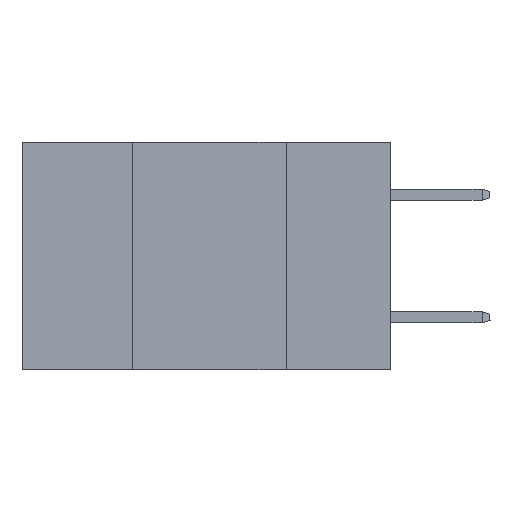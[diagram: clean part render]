
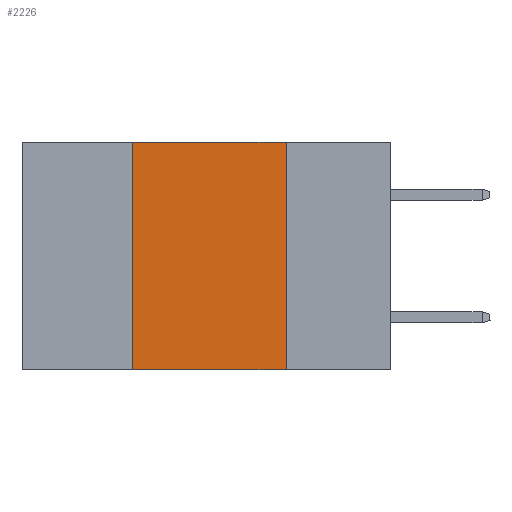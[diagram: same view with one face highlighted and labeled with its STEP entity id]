
A CAD part, left-side view. The second image highlights one B-rep face of the part: STEP entity #2226.
In plain terms, the highlighted planar face has unit normal (-1, 0, 0).
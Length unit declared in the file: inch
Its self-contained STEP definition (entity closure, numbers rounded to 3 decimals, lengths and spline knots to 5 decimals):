
#25 = DIRECTION ( 'NONE',  ( 0., 0., -1. ) ) ;
#101 = VERTEX_POINT ( 'NONE', #484 ) ;
#113 = VERTEX_POINT ( 'NONE', #12711 ) ;
#406 = EDGE_CURVE ( 'NONE', #113, #9413, #10536, .T. ) ;
#484 = CARTESIAN_POINT ( 'NONE',  ( 0., 0.42, -0.37 ) ) ;
#490 = DIRECTION ( 'NONE',  ( 0., 0., 1. ) ) ;
#513 = CARTESIAN_POINT ( 'NONE',  ( 0., 0.42, 0. ) ) ;
#1226 = VECTOR ( 'NONE', #4649, 39.37008 ) ;
#1314 = VECTOR ( 'NONE', #18355, 39.37008 ) ;
#2226 = ADVANCED_FACE ( 'NONE', ( #9738 ), #15655, .F. ) ;
#2980 = EDGE_CURVE ( 'NONE', #7673, #113, #4818, .T. ) ;
#3678 = CARTESIAN_POINT ( 'NONE',  ( 0., 0.6, -0.37 ) ) ;
#4121 = CARTESIAN_POINT ( 'NONE',  ( 0., 0.17, 0. ) ) ;
#4517 = CARTESIAN_POINT ( 'NONE',  ( 0., 0.17, -0.37 ) ) ;
#4649 = DIRECTION ( 'NONE',  ( 0., -1., 0. ) ) ;
#4818 = LINE ( 'NONE', #10713, #1226 ) ;
#5288 = EDGE_LOOP ( 'NONE', ( #19977, #6167, #11014, #10120 ) ) ;
#5918 = VECTOR ( 'NONE', #16476, 39.37008 ) ;
#6167 = ORIENTED_EDGE ( 'NONE', *, *, #2980, .F. ) ;
#7673 = VERTEX_POINT ( 'NONE', #513 ) ;
#7856 = DIRECTION ( 'NONE',  ( 1., 0., 0. ) ) ;
#7920 = CARTESIAN_POINT ( 'NONE',  ( 0., 0.6, 0. ) ) ;
#9349 = AXIS2_PLACEMENT_3D ( 'NONE', #7920, #7856, #25 ) ;
#9413 = VERTEX_POINT ( 'NONE', #4517 ) ;
#9419 = EDGE_CURVE ( 'NONE', #101, #7673, #17375, .T. ) ;
#9507 = CARTESIAN_POINT ( 'NONE',  ( 0., 0.42, 0. ) ) ;
#9738 = FACE_OUTER_BOUND ( 'NONE', #5288, .T. ) ;
#10120 = ORIENTED_EDGE ( 'NONE', *, *, #15979, .T. ) ;
#10536 = LINE ( 'NONE', #4121, #5918 ) ;
#10713 = CARTESIAN_POINT ( 'NONE',  ( 0., 0.6, 0. ) ) ;
#11014 = ORIENTED_EDGE ( 'NONE', *, *, #9419, .F. ) ;
#12219 = VECTOR ( 'NONE', #490, 39.37008 ) ;
#12711 = CARTESIAN_POINT ( 'NONE',  ( 0., 0.17, 0. ) ) ;
#13951 = LINE ( 'NONE', #3678, #1314 ) ;
#15655 = PLANE ( 'NONE',  #9349 ) ;
#15979 = EDGE_CURVE ( 'NONE', #101, #9413, #13951, .T. ) ;
#16476 = DIRECTION ( 'NONE',  ( 0., 0., -1. ) ) ;
#17375 = LINE ( 'NONE', #9507, #12219 ) ;
#18355 = DIRECTION ( 'NONE',  ( 0., -1., 0. ) ) ;
#19977 = ORIENTED_EDGE ( 'NONE', *, *, #406, .F. ) ;
